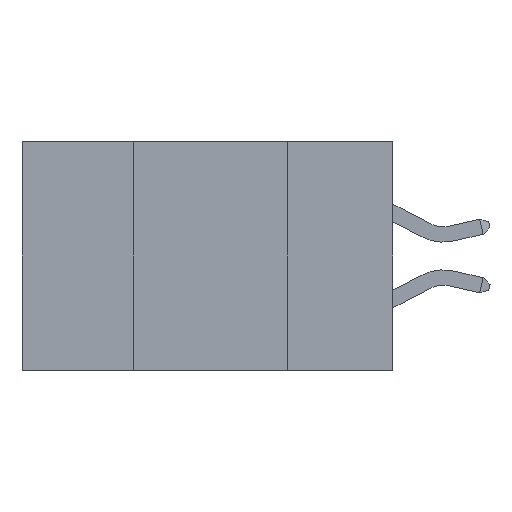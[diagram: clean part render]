
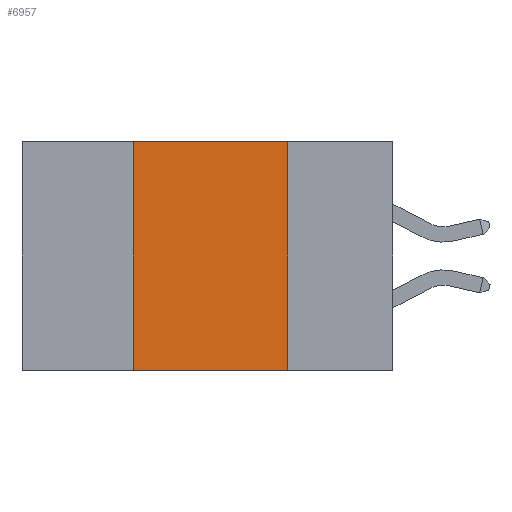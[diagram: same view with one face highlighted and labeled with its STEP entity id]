
A CAD part, left-side view. The second image highlights one B-rep face of the part: STEP entity #6957.
In plain terms, the highlighted planar face has unit normal (-1, 0, 0).
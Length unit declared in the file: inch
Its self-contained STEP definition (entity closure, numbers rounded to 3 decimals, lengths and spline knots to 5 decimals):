
#57 = VERTEX_POINT ( 'NONE', #1356 ) ;
#161 = DIRECTION ( 'NONE',  ( 0., -1., 0. ) ) ;
#923 = ORIENTED_EDGE ( 'NONE', *, *, #6968, .F. ) ;
#966 = ORIENTED_EDGE ( 'NONE', *, *, #4985, .T. ) ;
#1104 = VECTOR ( 'NONE', #3944, 39.37008 ) ;
#1356 = CARTESIAN_POINT ( 'NONE',  ( 0., 0.42, -0.37 ) ) ;
#1371 = CARTESIAN_POINT ( 'NONE',  ( 0., 0.6, 0. ) ) ;
#2394 = AXIS2_PLACEMENT_3D ( 'NONE', #1371, #7102, #5517 ) ;
#2477 = ORIENTED_EDGE ( 'NONE', *, *, #7489, .F. ) ;
#2661 = LINE ( 'NONE', #6288, #1104 ) ;
#2687 = CARTESIAN_POINT ( 'NONE',  ( 0., 0.6, -0.37 ) ) ;
#2754 = DIRECTION ( 'NONE',  ( 0., -1., 0. ) ) ;
#3172 = ORIENTED_EDGE ( 'NONE', *, *, #8502, .F. ) ;
#3944 = DIRECTION ( 'NONE',  ( 0., 0., 1. ) ) ;
#4266 = VERTEX_POINT ( 'NONE', #10301 ) ;
#4733 = VECTOR ( 'NONE', #161, 39.37008 ) ;
#4754 = VERTEX_POINT ( 'NONE', #9398 ) ;
#4985 = EDGE_CURVE ( 'NONE', #57, #4754, #5721, .T. ) ;
#5517 = DIRECTION ( 'NONE',  ( 0., 0., -1. ) ) ;
#5721 = LINE ( 'NONE', #2687, #6351 ) ;
#5729 = LINE ( 'NONE', #6083, #8411 ) ;
#6083 = CARTESIAN_POINT ( 'NONE',  ( 0., 0.17, 0. ) ) ;
#6288 = CARTESIAN_POINT ( 'NONE',  ( 0., 0.42, 0. ) ) ;
#6351 = VECTOR ( 'NONE', #2754, 39.37008 ) ;
#6361 = CARTESIAN_POINT ( 'NONE',  ( 0., 0.42, 0. ) ) ;
#6497 = FACE_OUTER_BOUND ( 'NONE', #8255, .T. ) ;
#6957 = ADVANCED_FACE ( 'NONE', ( #6497 ), #9333, .F. ) ;
#6968 = EDGE_CURVE ( 'NONE', #4266, #4754, #5729, .T. ) ;
#7102 = DIRECTION ( 'NONE',  ( 1., 0., 0. ) ) ;
#7131 = VERTEX_POINT ( 'NONE', #6361 ) ;
#7256 = LINE ( 'NONE', #9219, #4733 ) ;
#7489 = EDGE_CURVE ( 'NONE', #7131, #4266, #7256, .T. ) ;
#8255 = EDGE_LOOP ( 'NONE', ( #923, #2477, #3172, #966 ) ) ;
#8411 = VECTOR ( 'NONE', #9407, 39.37008 ) ;
#8502 = EDGE_CURVE ( 'NONE', #57, #7131, #2661, .T. ) ;
#9219 = CARTESIAN_POINT ( 'NONE',  ( 0., 0.6, 0. ) ) ;
#9333 = PLANE ( 'NONE',  #2394 ) ;
#9398 = CARTESIAN_POINT ( 'NONE',  ( 0., 0.17, -0.37 ) ) ;
#9407 = DIRECTION ( 'NONE',  ( 0., 0., -1. ) ) ;
#10301 = CARTESIAN_POINT ( 'NONE',  ( 0., 0.17, 0. ) ) ;
